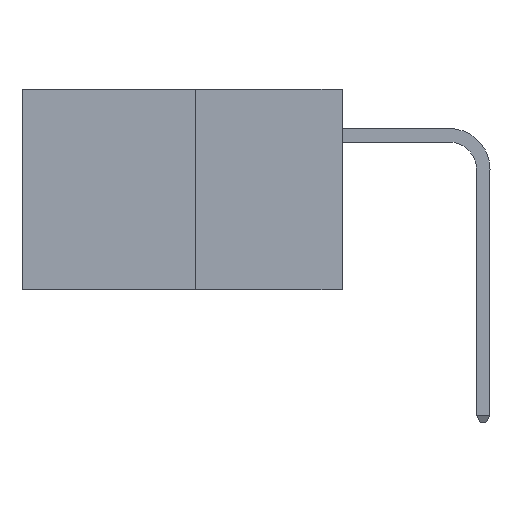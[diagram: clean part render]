
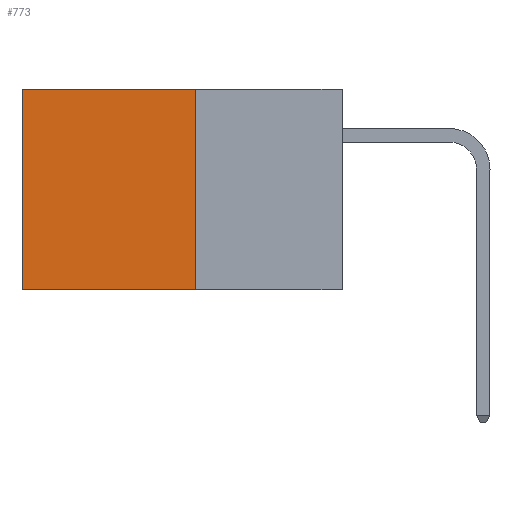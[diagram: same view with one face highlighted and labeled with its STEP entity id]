
A CAD part, left-side view. The second image highlights one B-rep face of the part: STEP entity #773.
In plain terms, the highlighted planar face has unit normal (-1, 0, 0).
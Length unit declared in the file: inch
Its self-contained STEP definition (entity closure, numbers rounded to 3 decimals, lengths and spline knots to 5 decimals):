
#773 = ADVANCED_FACE ( 'NONE', ( #10181 ), #16213, .F. ) ;
#1244 = AXIS2_PLACEMENT_3D ( 'NONE', #16382, #16051, #16322 ) ;
#1329 = CARTESIAN_POINT ( 'NONE',  ( 0.277, 0.59, -0.37 ) ) ;
#1726 = VECTOR ( 'NONE', #7763, 39.37008 ) ;
#2244 = CARTESIAN_POINT ( 'NONE',  ( 0.277, 0.59, 0. ) ) ;
#3135 = VERTEX_POINT ( 'NONE', #23337 ) ;
#3391 = VERTEX_POINT ( 'NONE', #2244 ) ;
#4189 = VECTOR ( 'NONE', #25045, 39.37008 ) ;
#4758 = DIRECTION ( 'NONE',  ( 0., 1., 0. ) ) ;
#5092 = CARTESIAN_POINT ( 'NONE',  ( 0.277, 0.27, -0.37 ) ) ;
#5144 = CARTESIAN_POINT ( 'NONE',  ( 0.277, 0.59, -0.37 ) ) ;
#5745 = VECTOR ( 'NONE', #4758, 39.37008 ) ;
#7763 = DIRECTION ( 'NONE',  ( 0., 1., 0. ) ) ;
#9180 = CARTESIAN_POINT ( 'NONE',  ( 0.277, 0.27, -0.37 ) ) ;
#9230 = VERTEX_POINT ( 'NONE', #1329 ) ;
#9813 = EDGE_LOOP ( 'NONE', ( #20189, #23092, #24435, #11913 ) ) ;
#10181 = FACE_OUTER_BOUND ( 'NONE', #9813, .T. ) ;
#11331 = CARTESIAN_POINT ( 'NONE',  ( 0.277, 0.27, -0.37 ) ) ;
#11913 = ORIENTED_EDGE ( 'NONE', *, *, #19714, .T. ) ;
#12762 = LINE ( 'NONE', #18824, #1726 ) ;
#13648 = EDGE_CURVE ( 'NONE', #13995, #9230, #28603, .T. ) ;
#13995 = VERTEX_POINT ( 'NONE', #11331 ) ;
#16051 = DIRECTION ( 'NONE',  ( 1., 0., 0. ) ) ;
#16128 = DIRECTION ( 'NONE',  ( 0., 0., -1. ) ) ;
#16213 = PLANE ( 'NONE',  #1244 ) ;
#16322 = DIRECTION ( 'NONE',  ( 0., 0., -1. ) ) ;
#16382 = CARTESIAN_POINT ( 'NONE',  ( 0.277, 0.27, -0.37 ) ) ;
#16864 = LINE ( 'NONE', #5092, #22016 ) ;
#18289 = EDGE_CURVE ( 'NONE', #3391, #9230, #27742, .T. ) ;
#18824 = CARTESIAN_POINT ( 'NONE',  ( 0.277, 0.27, 0. ) ) ;
#19714 = EDGE_CURVE ( 'NONE', #3135, #3391, #12762, .T. ) ;
#20189 = ORIENTED_EDGE ( 'NONE', *, *, #18289, .T. ) ;
#22016 = VECTOR ( 'NONE', #16128, 39.37008 ) ;
#23092 = ORIENTED_EDGE ( 'NONE', *, *, #13648, .F. ) ;
#23337 = CARTESIAN_POINT ( 'NONE',  ( 0.277, 0.27, 0. ) ) ;
#23620 = EDGE_CURVE ( 'NONE', #3135, #13995, #16864, .T. ) ;
#24435 = ORIENTED_EDGE ( 'NONE', *, *, #23620, .F. ) ;
#25045 = DIRECTION ( 'NONE',  ( 0., 0., -1. ) ) ;
#27742 = LINE ( 'NONE', #5144, #4189 ) ;
#28603 = LINE ( 'NONE', #9180, #5745 ) ;
